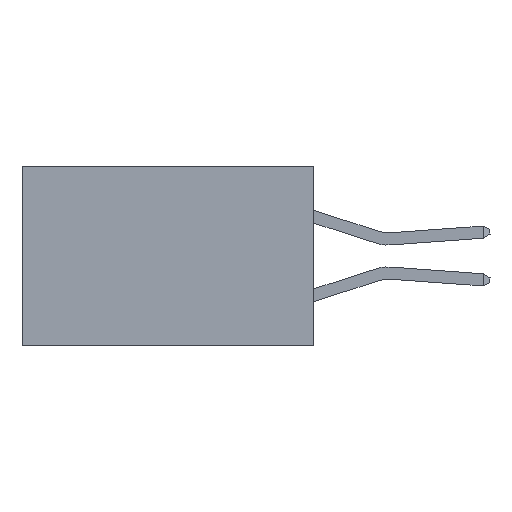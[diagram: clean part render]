
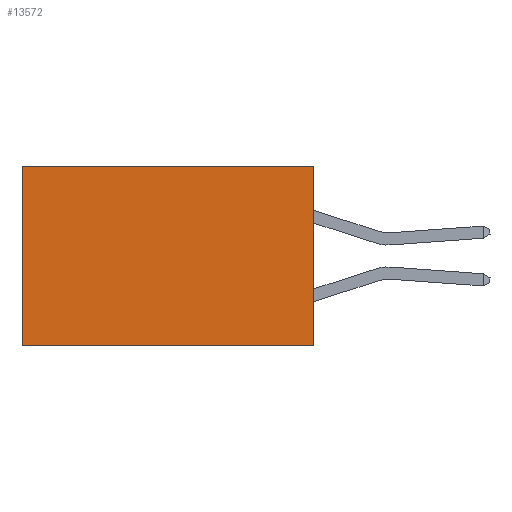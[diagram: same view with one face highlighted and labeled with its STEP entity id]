
A CAD part, left-side view. The second image highlights one B-rep face of the part: STEP entity #13572.
In plain terms, the highlighted planar face has unit normal (-1, 0, 0).
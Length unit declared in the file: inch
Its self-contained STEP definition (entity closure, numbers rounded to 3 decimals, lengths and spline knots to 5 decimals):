
#897 = CARTESIAN_POINT ( 'NONE',  ( 0.2875, 0.6, -0.37 ) ) ;
#1444 = ORIENTED_EDGE ( 'NONE', *, *, #26908, .T. ) ;
#3227 = CARTESIAN_POINT ( 'NONE',  ( 0.2875, 0., 0. ) ) ;
#4449 = ORIENTED_EDGE ( 'NONE', *, *, #32408, .F. ) ;
#5419 = EDGE_CURVE ( 'NONE', #7551, #22038, #21577, .T. ) ;
#7086 = PLANE ( 'NONE',  #23504 ) ;
#7148 = VECTOR ( 'NONE', #24553, 39.37008 ) ;
#7551 = VERTEX_POINT ( 'NONE', #20148 ) ;
#7578 = DIRECTION ( 'NONE',  ( 0., 0., -1. ) ) ;
#9305 = DIRECTION ( 'NONE',  ( 0., 1., 0. ) ) ;
#9665 = VECTOR ( 'NONE', #7578, 39.37008 ) ;
#12854 = CARTESIAN_POINT ( 'NONE',  ( 0.2875, 0., 0. ) ) ;
#13572 = ADVANCED_FACE ( 'NONE', ( #17147 ), #7086, .F. ) ;
#15096 = VECTOR ( 'NONE', #9305, 39.37008 ) ;
#16314 = DIRECTION ( 'NONE',  ( 0., 0., -1. ) ) ;
#17147 = FACE_OUTER_BOUND ( 'NONE', #27219, .T. ) ;
#18300 = CARTESIAN_POINT ( 'NONE',  ( 0.2875, 0., 0. ) ) ;
#18809 = ORIENTED_EDGE ( 'NONE', *, *, #5419, .T. ) ;
#19034 = VECTOR ( 'NONE', #16314, 39.37008 ) ;
#20148 = CARTESIAN_POINT ( 'NONE',  ( 0.2875, 0.6, 0. ) ) ;
#20338 = LINE ( 'NONE', #29537, #9665 ) ;
#21152 = DIRECTION ( 'NONE',  ( 1., 0., 0. ) ) ;
#21577 = LINE ( 'NONE', #27048, #19034 ) ;
#22038 = VERTEX_POINT ( 'NONE', #897 ) ;
#22900 = CARTESIAN_POINT ( 'NONE',  ( 0.2875, 0., -0.37 ) ) ;
#23194 = EDGE_CURVE ( 'NONE', #25533, #22038, #24910, .T. ) ;
#23504 = AXIS2_PLACEMENT_3D ( 'NONE', #18300, #21152, #32058 ) ;
#23707 = ORIENTED_EDGE ( 'NONE', *, *, #23194, .F. ) ;
#23791 = LINE ( 'NONE', #3227, #7148 ) ;
#24553 = DIRECTION ( 'NONE',  ( 0., 1., 0. ) ) ;
#24910 = LINE ( 'NONE', #22900, #15096 ) ;
#25533 = VERTEX_POINT ( 'NONE', #30015 ) ;
#26908 = EDGE_CURVE ( 'NONE', #29376, #7551, #23791, .T. ) ;
#27048 = CARTESIAN_POINT ( 'NONE',  ( 0.2875, 0.6, 0. ) ) ;
#27219 = EDGE_LOOP ( 'NONE', ( #18809, #23707, #4449, #1444 ) ) ;
#29376 = VERTEX_POINT ( 'NONE', #12854 ) ;
#29537 = CARTESIAN_POINT ( 'NONE',  ( 0.2875, 0., 0. ) ) ;
#30015 = CARTESIAN_POINT ( 'NONE',  ( 0.2875, 0., -0.37 ) ) ;
#32058 = DIRECTION ( 'NONE',  ( 0., 0., -1. ) ) ;
#32408 = EDGE_CURVE ( 'NONE', #29376, #25533, #20338, .T. ) ;
